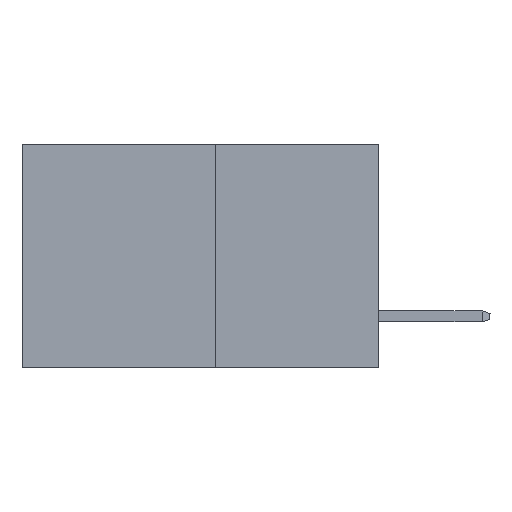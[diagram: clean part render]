
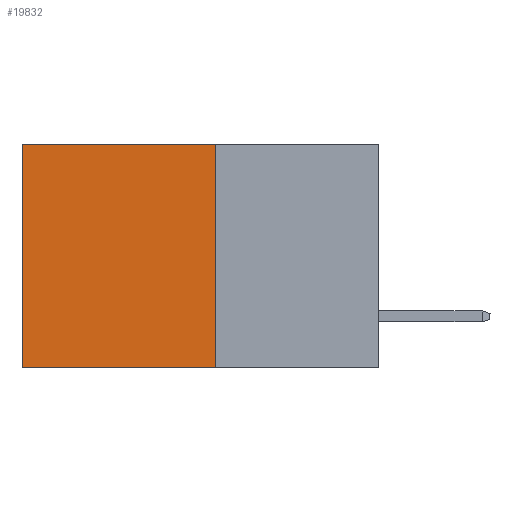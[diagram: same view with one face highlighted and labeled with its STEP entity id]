
A CAD part, left-side view. The second image highlights one B-rep face of the part: STEP entity #19832.
In plain terms, the highlighted planar face has unit normal (-1, 0, 0).
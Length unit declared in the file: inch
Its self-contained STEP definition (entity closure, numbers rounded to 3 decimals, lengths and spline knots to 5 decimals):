
#63 = CARTESIAN_POINT ( 'NONE',  ( 0.277, 0.27, -0.37 ) ) ;
#1381 = VERTEX_POINT ( 'NONE', #20610 ) ;
#1622 = VERTEX_POINT ( 'NONE', #63 ) ;
#2103 = DIRECTION ( 'NONE',  ( 0., 1., 0. ) ) ;
#2396 = VERTEX_POINT ( 'NONE', #17191 ) ;
#2575 = VERTEX_POINT ( 'NONE', #9933 ) ;
#2790 = DIRECTION ( 'NONE',  ( 1., 0., 0. ) ) ;
#4925 = CARTESIAN_POINT ( 'NONE',  ( 0.277, 0.27, -0.37 ) ) ;
#4963 = VECTOR ( 'NONE', #2103, 39.37008 ) ;
#6142 = AXIS2_PLACEMENT_3D ( 'NONE', #10814, #2790, #16818 ) ;
#6457 = ORIENTED_EDGE ( 'NONE', *, *, #24149, .F. ) ;
#6961 = DIRECTION ( 'NONE',  ( 0., 0., -1. ) ) ;
#7777 = EDGE_CURVE ( 'NONE', #1381, #2396, #15302, .T. ) ;
#8782 = PLANE ( 'NONE',  #6142 ) ;
#8786 = LINE ( 'NONE', #19913, #18735 ) ;
#8942 = FACE_OUTER_BOUND ( 'NONE', #16272, .T. ) ;
#9933 = CARTESIAN_POINT ( 'NONE',  ( 0.277, 0.27, 0. ) ) ;
#9969 = VECTOR ( 'NONE', #12598, 39.37008 ) ;
#10034 = DIRECTION ( 'NONE',  ( 0., 1., 0. ) ) ;
#10323 = LINE ( 'NONE', #21973, #4963 ) ;
#10566 = CARTESIAN_POINT ( 'NONE',  ( 0.277, 0.59, -0.37 ) ) ;
#10814 = CARTESIAN_POINT ( 'NONE',  ( 0.277, 0.27, -0.37 ) ) ;
#12357 = ORIENTED_EDGE ( 'NONE', *, *, #7777, .T. ) ;
#12598 = DIRECTION ( 'NONE',  ( 0., 0., -1. ) ) ;
#13670 = EDGE_CURVE ( 'NONE', #1622, #2396, #8786, .T. ) ;
#14656 = ORIENTED_EDGE ( 'NONE', *, *, #13670, .F. ) ;
#15302 = LINE ( 'NONE', #10566, #9969 ) ;
#15657 = LINE ( 'NONE', #4925, #20872 ) ;
#16272 = EDGE_LOOP ( 'NONE', ( #12357, #14656, #6457, #22463 ) ) ;
#16818 = DIRECTION ( 'NONE',  ( 0., 0., -1. ) ) ;
#17065 = EDGE_CURVE ( 'NONE', #2575, #1381, #10323, .T. ) ;
#17191 = CARTESIAN_POINT ( 'NONE',  ( 0.277, 0.59, -0.37 ) ) ;
#18735 = VECTOR ( 'NONE', #10034, 39.37008 ) ;
#19832 = ADVANCED_FACE ( 'NONE', ( #8942 ), #8782, .F. ) ;
#19913 = CARTESIAN_POINT ( 'NONE',  ( 0.277, 0.27, -0.37 ) ) ;
#20610 = CARTESIAN_POINT ( 'NONE',  ( 0.277, 0.59, 0. ) ) ;
#20872 = VECTOR ( 'NONE', #6961, 39.37008 ) ;
#21973 = CARTESIAN_POINT ( 'NONE',  ( 0.277, 0.27, 0. ) ) ;
#22463 = ORIENTED_EDGE ( 'NONE', *, *, #17065, .T. ) ;
#24149 = EDGE_CURVE ( 'NONE', #2575, #1622, #15657, .T. ) ;
